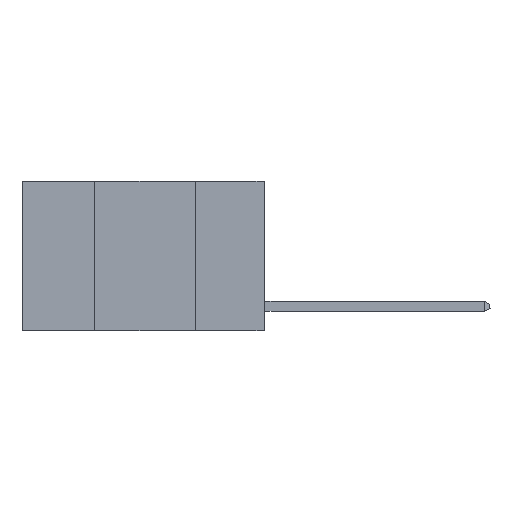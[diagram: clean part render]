
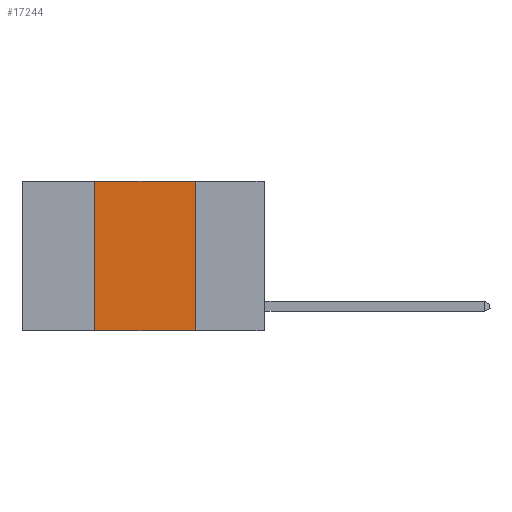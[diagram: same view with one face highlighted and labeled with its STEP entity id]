
A CAD part, left-side view. The second image highlights one B-rep face of the part: STEP entity #17244.
In plain terms, the highlighted planar face has unit normal (-1, 0, 0).
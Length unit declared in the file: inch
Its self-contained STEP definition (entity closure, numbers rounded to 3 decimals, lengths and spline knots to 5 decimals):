
#308 = EDGE_CURVE ( 'NONE', #13478, #1133, #11174, .T. ) ;
#331 = DIRECTION ( 'NONE',  ( 0., -1., 0. ) ) ;
#523 = EDGE_CURVE ( 'NONE', #16083, #1133, #2817, .T. ) ;
#726 = PLANE ( 'NONE',  #17679 ) ;
#1133 = VERTEX_POINT ( 'NONE', #6982 ) ;
#1616 = VECTOR ( 'NONE', #5673, 39.37008 ) ;
#1806 = ORIENTED_EDGE ( 'NONE', *, *, #308, .T. ) ;
#2249 = DIRECTION ( 'NONE',  ( 0., 0., -1. ) ) ;
#2382 = CARTESIAN_POINT ( 'NONE',  ( 0., 0.17, 0. ) ) ;
#2576 = LINE ( 'NONE', #4127, #1616 ) ;
#2817 = LINE ( 'NONE', #2382, #14451 ) ;
#3055 = VECTOR ( 'NONE', #331, 39.37008 ) ;
#4127 = CARTESIAN_POINT ( 'NONE',  ( 0., 0.6, 0. ) ) ;
#4786 = CARTESIAN_POINT ( 'NONE',  ( 0., 0.42, -0.37 ) ) ;
#5288 = CARTESIAN_POINT ( 'NONE',  ( 0., 0.6, 0. ) ) ;
#5673 = DIRECTION ( 'NONE',  ( 0., -1., 0. ) ) ;
#6063 = VECTOR ( 'NONE', #10549, 39.37008 ) ;
#6437 = EDGE_CURVE ( 'NONE', #18305, #16083, #2576, .T. ) ;
#6982 = CARTESIAN_POINT ( 'NONE',  ( 0., 0.17, -0.37 ) ) ;
#7955 = CARTESIAN_POINT ( 'NONE',  ( 0., 0.6, -0.37 ) ) ;
#10100 = LINE ( 'NONE', #18073, #6063 ) ;
#10549 = DIRECTION ( 'NONE',  ( 0., 0., 1. ) ) ;
#10602 = EDGE_LOOP ( 'NONE', ( #14972, #17016, #17476, #1806 ) ) ;
#10664 = FACE_OUTER_BOUND ( 'NONE', #10602, .T. ) ;
#11174 = LINE ( 'NONE', #7955, #3055 ) ;
#11381 = DIRECTION ( 'NONE',  ( 1., 0., 0. ) ) ;
#13226 = CARTESIAN_POINT ( 'NONE',  ( 0., 0.17, 0. ) ) ;
#13478 = VERTEX_POINT ( 'NONE', #4786 ) ;
#13963 = EDGE_CURVE ( 'NONE', #13478, #18305, #10100, .T. ) ;
#13987 = CARTESIAN_POINT ( 'NONE',  ( 0., 0.42, 0. ) ) ;
#14451 = VECTOR ( 'NONE', #17583, 39.37008 ) ;
#14972 = ORIENTED_EDGE ( 'NONE', *, *, #523, .F. ) ;
#16083 = VERTEX_POINT ( 'NONE', #13226 ) ;
#17016 = ORIENTED_EDGE ( 'NONE', *, *, #6437, .F. ) ;
#17244 = ADVANCED_FACE ( 'NONE', ( #10664 ), #726, .F. ) ;
#17476 = ORIENTED_EDGE ( 'NONE', *, *, #13963, .F. ) ;
#17583 = DIRECTION ( 'NONE',  ( 0., 0., -1. ) ) ;
#17679 = AXIS2_PLACEMENT_3D ( 'NONE', #5288, #11381, #2249 ) ;
#18073 = CARTESIAN_POINT ( 'NONE',  ( 0., 0.42, 0. ) ) ;
#18305 = VERTEX_POINT ( 'NONE', #13987 ) ;
